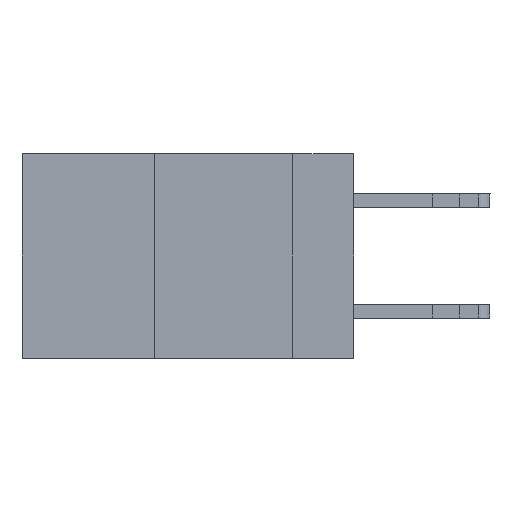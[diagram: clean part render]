
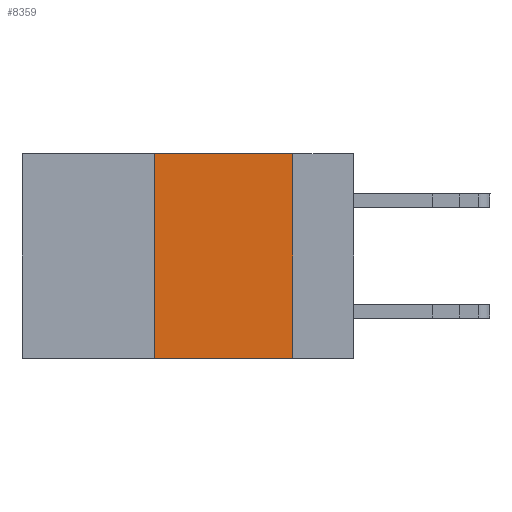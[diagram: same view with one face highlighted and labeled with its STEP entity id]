
A CAD part, left-side view. The second image highlights one B-rep face of the part: STEP entity #8359.
In plain terms, the highlighted planar face has unit normal (-1, 0, 0).
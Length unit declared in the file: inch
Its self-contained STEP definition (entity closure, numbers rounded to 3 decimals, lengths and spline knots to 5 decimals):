
#43 = CARTESIAN_POINT ( 'NONE',  ( 0., 0.6, 0. ) ) ;
#759 = LINE ( 'NONE', #19078, #1408 ) ;
#950 = CARTESIAN_POINT ( 'NONE',  ( 0., 0.6, -0.37 ) ) ;
#1408 = VECTOR ( 'NONE', #4607, 39.37008 ) ;
#1680 = VECTOR ( 'NONE', #19279, 39.37008 ) ;
#2329 = CARTESIAN_POINT ( 'NONE',  ( 0., 0.36, 0. ) ) ;
#3504 = ORIENTED_EDGE ( 'NONE', *, *, #7563, .F. ) ;
#4302 = VECTOR ( 'NONE', #9780, 39.37008 ) ;
#4328 = ORIENTED_EDGE ( 'NONE', *, *, #6720, .F. ) ;
#4607 = DIRECTION ( 'NONE',  ( 0., 0., -1. ) ) ;
#4913 = PLANE ( 'NONE',  #14588 ) ;
#5152 = LINE ( 'NONE', #11301, #4302 ) ;
#5288 = EDGE_CURVE ( 'NONE', #13215, #18665, #17400, .T. ) ;
#5706 = CARTESIAN_POINT ( 'NONE',  ( 0., 0.36, -0.37 ) ) ;
#6720 = EDGE_CURVE ( 'NONE', #8324, #18665, #759, .T. ) ;
#7419 = DIRECTION ( 'NONE',  ( 0., -1., 0. ) ) ;
#7563 = EDGE_CURVE ( 'NONE', #13215, #9705, #5152, .T. ) ;
#8324 = VERTEX_POINT ( 'NONE', #14165 ) ;
#8359 = ADVANCED_FACE ( 'NONE', ( #18855 ), #4913, .F. ) ;
#9705 = VERTEX_POINT ( 'NONE', #2329 ) ;
#9780 = DIRECTION ( 'NONE',  ( 0., 0., 1. ) ) ;
#10547 = LINE ( 'NONE', #43, #13126 ) ;
#11057 = DIRECTION ( 'NONE',  ( 1., 0., 0. ) ) ;
#11301 = CARTESIAN_POINT ( 'NONE',  ( 0., 0.36, 0. ) ) ;
#12274 = CARTESIAN_POINT ( 'NONE',  ( 0., 0.11, -0.37 ) ) ;
#13126 = VECTOR ( 'NONE', #7419, 39.37008 ) ;
#13215 = VERTEX_POINT ( 'NONE', #5706 ) ;
#13659 = EDGE_LOOP ( 'NONE', ( #4328, #17143, #3504, #19566 ) ) ;
#14165 = CARTESIAN_POINT ( 'NONE',  ( 0., 0.11, 0. ) ) ;
#14364 = CARTESIAN_POINT ( 'NONE',  ( 0., 0.6, 0. ) ) ;
#14588 = AXIS2_PLACEMENT_3D ( 'NONE', #14364, #11057, #17181 ) ;
#16792 = EDGE_CURVE ( 'NONE', #9705, #8324, #10547, .T. ) ;
#17143 = ORIENTED_EDGE ( 'NONE', *, *, #16792, .F. ) ;
#17181 = DIRECTION ( 'NONE',  ( 0., 0., -1. ) ) ;
#17400 = LINE ( 'NONE', #950, #1680 ) ;
#18665 = VERTEX_POINT ( 'NONE', #12274 ) ;
#18855 = FACE_OUTER_BOUND ( 'NONE', #13659, .T. ) ;
#19078 = CARTESIAN_POINT ( 'NONE',  ( 0., 0.11, 0. ) ) ;
#19279 = DIRECTION ( 'NONE',  ( 0., -1., 0. ) ) ;
#19566 = ORIENTED_EDGE ( 'NONE', *, *, #5288, .T. ) ;
